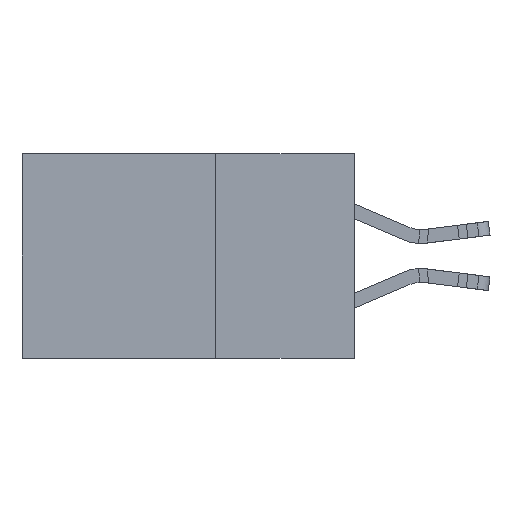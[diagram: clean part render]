
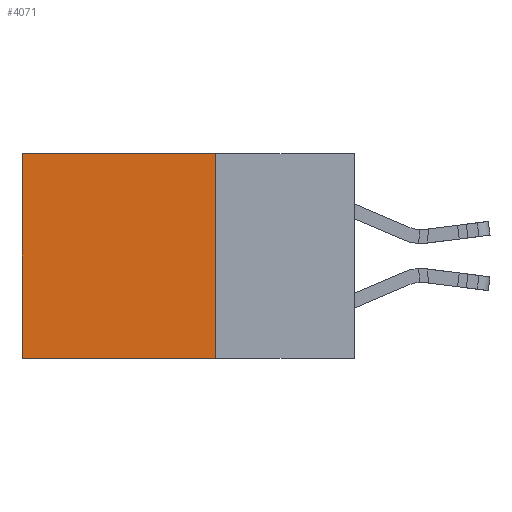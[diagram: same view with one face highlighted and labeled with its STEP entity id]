
A CAD part, left-side view. The second image highlights one B-rep face of the part: STEP entity #4071.
In plain terms, the highlighted planar face has unit normal (-1, 0, 0).
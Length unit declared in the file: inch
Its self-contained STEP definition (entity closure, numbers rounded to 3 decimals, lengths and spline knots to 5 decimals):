
#230 = ORIENTED_EDGE ( 'NONE', *, *, #3251, .F. ) ;
#2186 = DIRECTION ( 'NONE',  ( 0., 1., 0. ) ) ;
#2564 = CARTESIAN_POINT ( 'NONE',  ( 0.298, 0.25, 0. ) ) ;
#2950 = DIRECTION ( 'NONE',  ( 1., 0., 0. ) ) ;
#3140 = PLANE ( 'NONE',  #5383 ) ;
#3251 = EDGE_CURVE ( 'NONE', #18158, #4200, #10718, .T. ) ;
#3718 = DIRECTION ( 'NONE',  ( 0., 0., -1. ) ) ;
#4071 = ADVANCED_FACE ( 'NONE', ( #10702 ), #3140, .F. ) ;
#4200 = VERTEX_POINT ( 'NONE', #13046 ) ;
#5176 = EDGE_CURVE ( 'NONE', #19150, #4200, #21514, .T. ) ;
#5383 = AXIS2_PLACEMENT_3D ( 'NONE', #24780, #2950, #20641 ) ;
#8959 = EDGE_CURVE ( 'NONE', #10297, #19150, #15601, .T. ) ;
#10297 = VERTEX_POINT ( 'NONE', #23106 ) ;
#10545 = VECTOR ( 'NONE', #3718, 39.37008 ) ;
#10702 = FACE_OUTER_BOUND ( 'NONE', #25956, .T. ) ;
#10718 = LINE ( 'NONE', #15863, #26861 ) ;
#10926 = CARTESIAN_POINT ( 'NONE',  ( 0.298, 0.25, -0.37 ) ) ;
#12015 = CARTESIAN_POINT ( 'NONE',  ( 0.298, 0.6, 0. ) ) ;
#13046 = CARTESIAN_POINT ( 'NONE',  ( 0.298, 0.6, -0.37 ) ) ;
#13199 = LINE ( 'NONE', #24610, #25598 ) ;
#13918 = VECTOR ( 'NONE', #2186, 39.37008 ) ;
#14119 = ORIENTED_EDGE ( 'NONE', *, *, #8959, .T. ) ;
#14258 = ORIENTED_EDGE ( 'NONE', *, *, #5176, .T. ) ;
#15601 = LINE ( 'NONE', #2564, #13918 ) ;
#15863 = CARTESIAN_POINT ( 'NONE',  ( 0.298, 0.25, -0.37 ) ) ;
#16735 = CARTESIAN_POINT ( 'NONE',  ( 0.298, 0.6, 0. ) ) ;
#18158 = VERTEX_POINT ( 'NONE', #10926 ) ;
#18717 = EDGE_CURVE ( 'NONE', #10297, #18158, #13199, .T. ) ;
#19150 = VERTEX_POINT ( 'NONE', #12015 ) ;
#19719 = ORIENTED_EDGE ( 'NONE', *, *, #18717, .F. ) ;
#20641 = DIRECTION ( 'NONE',  ( 0., 0., -1. ) ) ;
#21514 = LINE ( 'NONE', #16735, #10545 ) ;
#22897 = DIRECTION ( 'NONE',  ( 0., 1., 0. ) ) ;
#23106 = CARTESIAN_POINT ( 'NONE',  ( 0.298, 0.25, 0. ) ) ;
#24610 = CARTESIAN_POINT ( 'NONE',  ( 0.298, 0.25, 0. ) ) ;
#24780 = CARTESIAN_POINT ( 'NONE',  ( 0.298, 0.25, 0. ) ) ;
#25598 = VECTOR ( 'NONE', #26524, 39.37008 ) ;
#25956 = EDGE_LOOP ( 'NONE', ( #14258, #230, #19719, #14119 ) ) ;
#26524 = DIRECTION ( 'NONE',  ( 0., 0., -1. ) ) ;
#26861 = VECTOR ( 'NONE', #22897, 39.37008 ) ;
